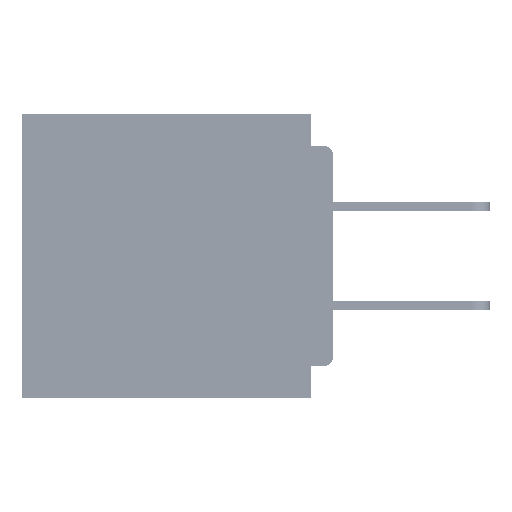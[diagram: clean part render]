
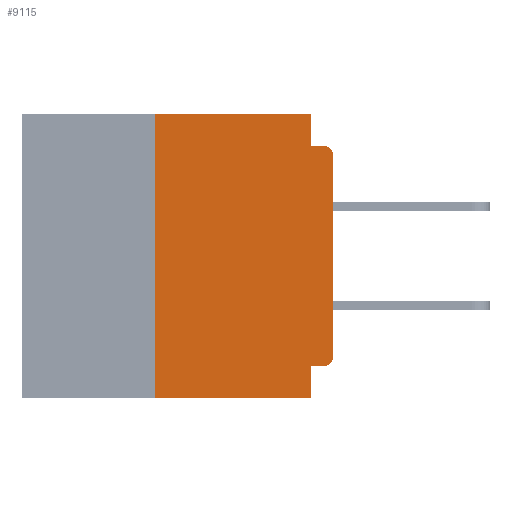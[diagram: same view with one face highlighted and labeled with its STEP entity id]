
A CAD part, left-side view. The second image highlights one B-rep face of the part: STEP entity #9115.
In plain terms, the highlighted planar face has unit normal (-1, 0, 0).
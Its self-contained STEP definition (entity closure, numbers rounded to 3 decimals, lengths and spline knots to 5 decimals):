
#363 = VECTOR ( 'NONE', #36615, 39.37008 ) ;
#522 = VERTEX_POINT ( 'NONE', #64854 ) ;
#2191 = VECTOR ( 'NONE', #25314, 39.37008 ) ;
#3474 = LINE ( 'NONE', #58618, #29782 ) ;
#4607 = CARTESIAN_POINT ( 'NONE',  ( 0., 0.031, -0.045 ) ) ;
#4906 = VERTEX_POINT ( 'NONE', #7590 ) ;
#4922 = CARTESIAN_POINT ( 'NONE',  ( 0., 0., -0.06 ) ) ;
#5629 = LINE ( 'NONE', #16110, #59943 ) ;
#6189 = VERTEX_POINT ( 'NONE', #23295 ) ;
#6847 = ORIENTED_EDGE ( 'NONE', *, *, #50588, .T. ) ;
#7590 = CARTESIAN_POINT ( 'NONE',  ( 0., 0.25, -0.4 ) ) ;
#8297 = EDGE_CURVE ( 'NONE', #47897, #34348, #5629, .T. ) ;
#9115 = ADVANCED_FACE ( 'NONE', ( #26992 ), #11878, .F. ) ;
#9318 = ORIENTED_EDGE ( 'NONE', *, *, #63603, .T. ) ;
#10127 = CARTESIAN_POINT ( 'NONE',  ( 0., 0.437, 0. ) ) ;
#11878 = PLANE ( 'NONE',  #14754 ) ;
#12395 = CARTESIAN_POINT ( 'NONE',  ( 0., 0.031, -0.4 ) ) ;
#13490 = CARTESIAN_POINT ( 'NONE',  ( 0., 0.015, -0.06 ) ) ;
#14317 = LINE ( 'NONE', #10127, #363 ) ;
#14754 = AXIS2_PLACEMENT_3D ( 'NONE', #16942, #48792, #17164 ) ;
#15527 = DIRECTION ( 'NONE',  ( 0., 0., 1. ) ) ;
#15915 = ORIENTED_EDGE ( 'NONE', *, *, #54810, .F. ) ;
#16110 = CARTESIAN_POINT ( 'NONE',  ( 0., 0., -0.355 ) ) ;
#16238 = VECTOR ( 'NONE', #15527, 39.37008 ) ;
#16942 = CARTESIAN_POINT ( 'NONE',  ( 0., 0.437, 0. ) ) ;
#17164 = DIRECTION ( 'NONE',  ( 0., 0., -1. ) ) ;
#17819 = LINE ( 'NONE', #20023, #2191 ) ;
#17850 = VECTOR ( 'NONE', #50472, 39.37008 ) ;
#18799 = DIRECTION ( 'NONE',  ( 0., 0., -1. ) ) ;
#19317 = CARTESIAN_POINT ( 'NONE',  ( 0., 0.031, -0.4 ) ) ;
#20023 = CARTESIAN_POINT ( 'NONE',  ( 0., 0.437, -0.4 ) ) ;
#21974 = CARTESIAN_POINT ( 'NONE',  ( 0., 0.031, -0.355 ) ) ;
#23295 = CARTESIAN_POINT ( 'NONE',  ( 0., 0., -0.34 ) ) ;
#24327 = CARTESIAN_POINT ( 'NONE',  ( 0., 0.015, -0.34 ) ) ;
#24768 = EDGE_LOOP ( 'NONE', ( #9318, #42022, #42809, #61266, #42667, #15915, #6847, #28793, #44623, #60333 ) ) ;
#25314 = DIRECTION ( 'NONE',  ( 0., -1., 0. ) ) ;
#26904 = EDGE_CURVE ( 'NONE', #47897, #6189, #33788, .T. ) ;
#26992 = FACE_OUTER_BOUND ( 'NONE', #24768, .T. ) ;
#28441 = CARTESIAN_POINT ( 'NONE',  ( 0., 0.015, -0.045 ) ) ;
#28793 = ORIENTED_EDGE ( 'NONE', *, *, #32132, .F. ) ;
#29612 = DIRECTION ( 'NONE',  ( 0., 0., -1. ) ) ;
#29782 = VECTOR ( 'NONE', #32360, 39.37008 ) ;
#31834 = LINE ( 'NONE', #60742, #17850 ) ;
#32132 = EDGE_CURVE ( 'NONE', #34348, #41456, #38334, .T. ) ;
#32360 = DIRECTION ( 'NONE',  ( 0., 0., -1. ) ) ;
#33788 = CIRCLE ( 'NONE', #55903, 0.015 ) ;
#34348 = VERTEX_POINT ( 'NONE', #21974 ) ;
#35961 = CARTESIAN_POINT ( 'NONE',  ( 0., 0.031, 0. ) ) ;
#36615 = DIRECTION ( 'NONE',  ( 0., -1., 0. ) ) ;
#38334 = LINE ( 'NONE', #12395, #49062 ) ;
#41456 = VERTEX_POINT ( 'NONE', #19317 ) ;
#42022 = ORIENTED_EDGE ( 'NONE', *, *, #61034, .T. ) ;
#42207 = VERTEX_POINT ( 'NONE', #4922 ) ;
#42667 = ORIENTED_EDGE ( 'NONE', *, *, #52564, .F. ) ;
#42687 = DIRECTION ( 'NONE',  ( 0., 1., 0. ) ) ;
#42696 = LINE ( 'NONE', #52435, #16238 ) ;
#42809 = ORIENTED_EDGE ( 'NONE', *, *, #46555, .F. ) ;
#44623 = ORIENTED_EDGE ( 'NONE', *, *, #8297, .F. ) ;
#44748 = VECTOR ( 'NONE', #52188, 39.37008 ) ;
#45142 = VERTEX_POINT ( 'NONE', #35961 ) ;
#45912 = VERTEX_POINT ( 'NONE', #4607 ) ;
#46379 = LINE ( 'NONE', #46925, #44748 ) ;
#46436 = AXIS2_PLACEMENT_3D ( 'NONE', #13490, #50407, #18799 ) ;
#46555 = EDGE_CURVE ( 'NONE', #45912, #64105, #46379, .T. ) ;
#46925 = CARTESIAN_POINT ( 'NONE',  ( 0., 0., -0.045 ) ) ;
#47897 = VERTEX_POINT ( 'NONE', #59097 ) ;
#48792 = DIRECTION ( 'NONE',  ( 1., 0., 0. ) ) ;
#49062 = VECTOR ( 'NONE', #49304, 39.37008 ) ;
#49304 = DIRECTION ( 'NONE',  ( 0., 0., -1. ) ) ;
#50407 = DIRECTION ( 'NONE',  ( -1., 0., 0. ) ) ;
#50472 = DIRECTION ( 'NONE',  ( 0., 0., 1. ) ) ;
#50588 = EDGE_CURVE ( 'NONE', #4906, #41456, #17819, .T. ) ;
#52188 = DIRECTION ( 'NONE',  ( 0., -1., 0. ) ) ;
#52435 = CARTESIAN_POINT ( 'NONE',  ( 0., 0.25, -0.4 ) ) ;
#52564 = EDGE_CURVE ( 'NONE', #522, #45142, #14317, .T. ) ;
#54810 = EDGE_CURVE ( 'NONE', #4906, #522, #42696, .T. ) ;
#55903 = AXIS2_PLACEMENT_3D ( 'NONE', #24327, #61145, #29612 ) ;
#58587 = EDGE_CURVE ( 'NONE', #45142, #45912, #3474, .T. ) ;
#58608 = CIRCLE ( 'NONE', #46436, 0.015 ) ;
#58618 = CARTESIAN_POINT ( 'NONE',  ( 0., 0.031, 0. ) ) ;
#59097 = CARTESIAN_POINT ( 'NONE',  ( 0., 0.015, -0.355 ) ) ;
#59943 = VECTOR ( 'NONE', #42687, 39.37008 ) ;
#60333 = ORIENTED_EDGE ( 'NONE', *, *, #26904, .T. ) ;
#60742 = CARTESIAN_POINT ( 'NONE',  ( 0., 0., 0. ) ) ;
#61034 = EDGE_CURVE ( 'NONE', #42207, #64105, #58608, .T. ) ;
#61145 = DIRECTION ( 'NONE',  ( -1., 0., 0. ) ) ;
#61266 = ORIENTED_EDGE ( 'NONE', *, *, #58587, .F. ) ;
#63603 = EDGE_CURVE ( 'NONE', #6189, #42207, #31834, .T. ) ;
#64105 = VERTEX_POINT ( 'NONE', #28441 ) ;
#64854 = CARTESIAN_POINT ( 'NONE',  ( 0., 0.25, 0. ) ) ;
